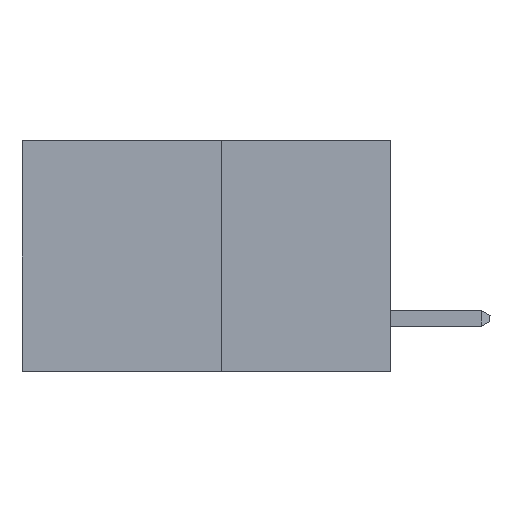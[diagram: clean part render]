
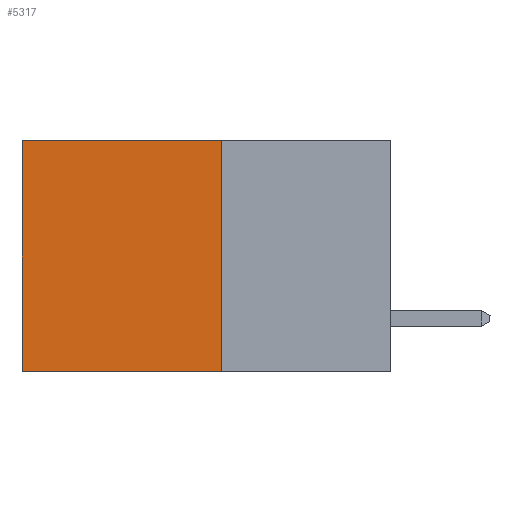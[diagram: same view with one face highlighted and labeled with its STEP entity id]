
A CAD part, left-side view. The second image highlights one B-rep face of the part: STEP entity #5317.
In plain terms, the highlighted planar face has unit normal (-1, 0, 0).
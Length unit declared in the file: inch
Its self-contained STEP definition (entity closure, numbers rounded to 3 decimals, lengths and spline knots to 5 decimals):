
#49 = CARTESIAN_POINT ( 'NONE',  ( 0.277, 0.27, -0.37 ) ) ;
#130 = CARTESIAN_POINT ( 'NONE',  ( 0.277, 0.59, 0. ) ) ;
#550 = LINE ( 'NONE', #49, #5433 ) ;
#741 = ORIENTED_EDGE ( 'NONE', *, *, #9561, .F. ) ;
#1231 = CARTESIAN_POINT ( 'NONE',  ( 0.277, 0.59, -0.37 ) ) ;
#1271 = CARTESIAN_POINT ( 'NONE',  ( 0.277, 0.27, 0. ) ) ;
#1447 = DIRECTION ( 'NONE',  ( 0., 0., -1. ) ) ;
#1940 = LINE ( 'NONE', #7303, #11428 ) ;
#3207 = FACE_OUTER_BOUND ( 'NONE', #11957, .T. ) ;
#3354 = PLANE ( 'NONE',  #4590 ) ;
#3900 = EDGE_CURVE ( 'NONE', #6593, #12332, #10674, .T. ) ;
#3944 = DIRECTION ( 'NONE',  ( 0., 1., 0. ) ) ;
#4036 = EDGE_CURVE ( 'NONE', #6593, #10656, #1940, .T. ) ;
#4265 = ORIENTED_EDGE ( 'NONE', *, *, #3900, .T. ) ;
#4339 = DIRECTION ( 'NONE',  ( 0., 0., -1. ) ) ;
#4590 = AXIS2_PLACEMENT_3D ( 'NONE', #8217, #10202, #4339 ) ;
#4688 = LINE ( 'NONE', #10777, #9313 ) ;
#5317 = ADVANCED_FACE ( 'NONE', ( #3207 ), #3354, .F. ) ;
#5433 = VECTOR ( 'NONE', #3944, 39.37008 ) ;
#6258 = ORIENTED_EDGE ( 'NONE', *, *, #4036, .F. ) ;
#6399 = ORIENTED_EDGE ( 'NONE', *, *, #8611, .T. ) ;
#6593 = VERTEX_POINT ( 'NONE', #9851 ) ;
#6889 = DIRECTION ( 'NONE',  ( 0., 0., -1. ) ) ;
#7303 = CARTESIAN_POINT ( 'NONE',  ( 0.277, 0.27, -0.37 ) ) ;
#8137 = DIRECTION ( 'NONE',  ( 0., 1., 0. ) ) ;
#8217 = CARTESIAN_POINT ( 'NONE',  ( 0.277, 0.27, -0.37 ) ) ;
#8418 = VECTOR ( 'NONE', #8137, 39.37008 ) ;
#8611 = EDGE_CURVE ( 'NONE', #12332, #11145, #4688, .T. ) ;
#9313 = VECTOR ( 'NONE', #6889, 39.37008 ) ;
#9561 = EDGE_CURVE ( 'NONE', #10656, #11145, #550, .T. ) ;
#9851 = CARTESIAN_POINT ( 'NONE',  ( 0.277, 0.27, 0. ) ) ;
#10202 = DIRECTION ( 'NONE',  ( 1., 0., 0. ) ) ;
#10656 = VERTEX_POINT ( 'NONE', #11281 ) ;
#10674 = LINE ( 'NONE', #1271, #8418 ) ;
#10777 = CARTESIAN_POINT ( 'NONE',  ( 0.277, 0.59, -0.37 ) ) ;
#11145 = VERTEX_POINT ( 'NONE', #1231 ) ;
#11281 = CARTESIAN_POINT ( 'NONE',  ( 0.277, 0.27, -0.37 ) ) ;
#11428 = VECTOR ( 'NONE', #1447, 39.37008 ) ;
#11957 = EDGE_LOOP ( 'NONE', ( #6399, #741, #6258, #4265 ) ) ;
#12332 = VERTEX_POINT ( 'NONE', #130 ) ;
